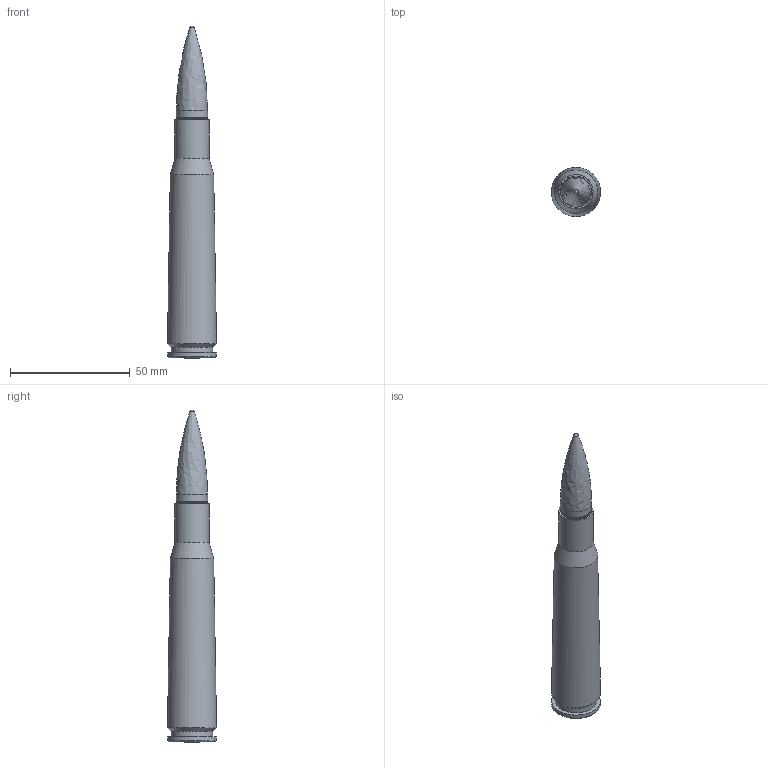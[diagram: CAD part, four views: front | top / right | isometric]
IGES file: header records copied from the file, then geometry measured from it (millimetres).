
Global section: file name: 50bmg_assem; native system: Autodesk Inventor 2017; preprocessor: unknown; author: user; date: 20201107.114035; units: millimetre
Bounding box: 20.46 x 20.47 x 138.41 mm (x, y, z)
Volume: 13163 mm3; surface area: 13437.2 mm2
Topology: 4 solids, 4 shells, 309 faces, 913 edges, 613 vertices
Faces by surface type: bspline 309
